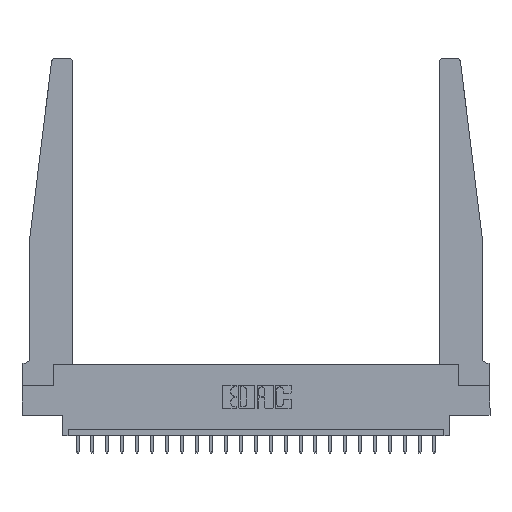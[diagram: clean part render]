
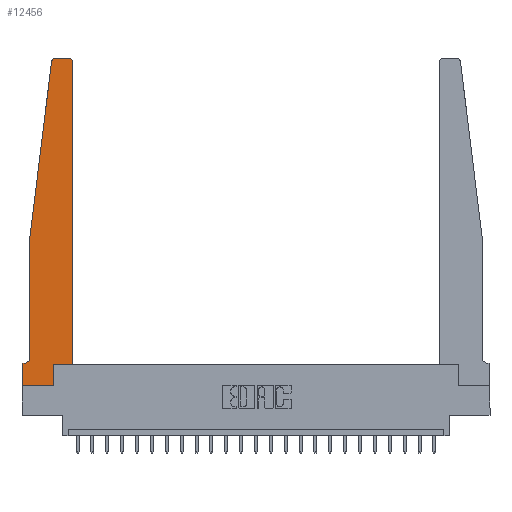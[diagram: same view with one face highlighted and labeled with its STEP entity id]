
A CAD part, top view. The second image highlights one B-rep face of the part: STEP entity #12456.
In plain terms, the highlighted planar face has unit normal (0, 0, 1).
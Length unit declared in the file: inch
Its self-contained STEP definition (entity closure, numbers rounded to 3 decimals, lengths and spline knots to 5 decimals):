
#195 = DIRECTION ( 'NONE',  ( 1., 0., 0. ) ) ;
#220 = CARTESIAN_POINT ( 'NONE',  ( 0.2605, 0.18, 0.37 ) ) ;
#1024 = VECTOR ( 'NONE', #21751, 39.37008 ) ;
#1156 = VECTOR ( 'NONE', #7244, 39.37008 ) ;
#1411 = VECTOR ( 'NONE', #16611, 39.37008 ) ;
#1470 = VERTEX_POINT ( 'NONE', #17604 ) ;
#1848 = DIRECTION ( 'NONE',  ( 0., 1., 0. ) ) ;
#1946 = LINE ( 'NONE', #5581, #20961 ) ;
#2087 = LINE ( 'NONE', #2330, #1411 ) ;
#2330 = CARTESIAN_POINT ( 'NONE',  ( 0.065, 0.1875, 0.37 ) ) ;
#2447 = CARTESIAN_POINT ( 'NONE',  ( 0., 0.1875, 0.37 ) ) ;
#2589 = ORIENTED_EDGE ( 'NONE', *, *, #8702, .T. ) ;
#2683 = VECTOR ( 'NONE', #5161, 39.37008 ) ;
#3617 = ORIENTED_EDGE ( 'NONE', *, *, #18605, .T. ) ;
#3707 = ORIENTED_EDGE ( 'NONE', *, *, #18947, .T. ) ;
#4768 = LINE ( 'NONE', #8746, #23114 ) ;
#5161 = DIRECTION ( 'NONE',  ( 0., -1., 0. ) ) ;
#5249 = CARTESIAN_POINT ( 'NONE',  ( 0., 0.1875, 0.37 ) ) ;
#5581 = CARTESIAN_POINT ( 'NONE',  ( 0.065, 1.25, 0.37 ) ) ;
#5660 = AXIS2_PLACEMENT_3D ( 'NONE', #9316, #14349, #16455 ) ;
#5969 = CIRCLE ( 'NONE', #7462, 0.03 ) ;
#6308 = CARTESIAN_POINT ( 'NONE',  ( 0.395, 2.75, 0.37 ) ) ;
#6386 = EDGE_CURVE ( 'NONE', #6647, #10797, #18316, .T. ) ;
#6418 = CARTESIAN_POINT ( 'NONE',  ( 0., 0., 0.37 ) ) ;
#6507 = DIRECTION ( 'NONE',  ( 0., 0., -1. ) ) ;
#6519 = DIRECTION ( 'NONE',  ( 1., 0., 0. ) ) ;
#6593 = CARTESIAN_POINT ( 'NONE',  ( 0.065, 1.25, 0.37 ) ) ;
#6647 = VERTEX_POINT ( 'NONE', #15839 ) ;
#6669 = ORIENTED_EDGE ( 'NONE', *, *, #12583, .T. ) ;
#7029 = EDGE_CURVE ( 'NONE', #15122, #15723, #5969, .T. ) ;
#7244 = DIRECTION ( 'NONE',  ( -1., 0., 0. ) ) ;
#7292 = CARTESIAN_POINT ( 'NONE',  ( 0.015, 0.1875, 0.37 ) ) ;
#7462 = AXIS2_PLACEMENT_3D ( 'NONE', #21162, #21394, #195 ) ;
#7508 = ORIENTED_EDGE ( 'NONE', *, *, #15579, .T. ) ;
#7677 = CARTESIAN_POINT ( 'NONE',  ( 0.2605, 0.18, 0.37 ) ) ;
#7858 = ORIENTED_EDGE ( 'NONE', *, *, #16598, .T. ) ;
#8171 = DIRECTION ( 'NONE',  ( -1., 0., 0. ) ) ;
#8194 = LINE ( 'NONE', #6418, #22127 ) ;
#8702 = EDGE_CURVE ( 'NONE', #14537, #20642, #16121, .T. ) ;
#8746 = CARTESIAN_POINT ( 'NONE',  ( 0.425, 0.18, 0.37 ) ) ;
#9017 = ORIENTED_EDGE ( 'NONE', *, *, #17111, .T. ) ;
#9165 = CARTESIAN_POINT ( 'NONE',  ( 0.27653, 2.75, 0.37 ) ) ;
#9316 = CARTESIAN_POINT ( 'NONE',  ( 0.395, 2.72, 0.37 ) ) ;
#9418 = DIRECTION ( 'NONE',  ( 0., 1., 0. ) ) ;
#9622 = CARTESIAN_POINT ( 'NONE',  ( 0.2605, 0., 0.37 ) ) ;
#9676 = VERTEX_POINT ( 'NONE', #6308 ) ;
#10520 = CIRCLE ( 'NONE', #5660, 0.03 ) ;
#10556 = CARTESIAN_POINT ( 'NONE',  ( 0.065, 1.25, 0.37 ) ) ;
#10649 = DIRECTION ( 'NONE',  ( 1., 0., 0. ) ) ;
#10797 = VERTEX_POINT ( 'NONE', #10815 ) ;
#10815 = CARTESIAN_POINT ( 'NONE',  ( 0.425, 2.72, 0.37 ) ) ;
#10895 = CARTESIAN_POINT ( 'NONE',  ( 0.25, 2.75, 0.37 ) ) ;
#10896 = CIRCLE ( 'NONE', #16109, 0.05 ) ;
#10981 = DIRECTION ( 'NONE',  ( -0.122, -0.992, 0. ) ) ;
#12015 = CARTESIAN_POINT ( 'NONE',  ( 0., 0., 0.37 ) ) ;
#12417 = DIRECTION ( 'NONE',  ( 0., 0., 1. ) ) ;
#12456 = ADVANCED_FACE ( 'NONE', ( #23060 ), #19537, .T. ) ;
#12573 = EDGE_CURVE ( 'NONE', #20124, #21087, #2087, .T. ) ;
#12583 = EDGE_CURVE ( 'NONE', #20642, #18800, #16260, .T. ) ;
#12707 = CARTESIAN_POINT ( 'NONE',  ( 0.425, 0.18, 0.37 ) ) ;
#12746 = CARTESIAN_POINT ( 'NONE',  ( 0., 0., 0.37 ) ) ;
#12835 = EDGE_CURVE ( 'NONE', #18800, #6647, #4768, .T. ) ;
#14349 = DIRECTION ( 'NONE',  ( 0., 0., 1. ) ) ;
#14537 = VERTEX_POINT ( 'NONE', #12015 ) ;
#15122 = VERTEX_POINT ( 'NONE', #9165 ) ;
#15149 = ORIENTED_EDGE ( 'NONE', *, *, #7029, .T. ) ;
#15181 = ORIENTED_EDGE ( 'NONE', *, *, #17052, .T. ) ;
#15251 = VECTOR ( 'NONE', #9418, 39.37008 ) ;
#15428 = CARTESIAN_POINT ( 'NONE',  ( 0.015, 0.2375, 0.37 ) ) ;
#15579 = EDGE_CURVE ( 'NONE', #15723, #17374, #1946, .T. ) ;
#15723 = VERTEX_POINT ( 'NONE', #17175 ) ;
#15839 = CARTESIAN_POINT ( 'NONE',  ( 0.425, 0.18, 0.37 ) ) ;
#16109 = AXIS2_PLACEMENT_3D ( 'NONE', #15428, #6507, #8171 ) ;
#16121 = LINE ( 'NONE', #12746, #1024 ) ;
#16260 = LINE ( 'NONE', #220, #21977 ) ;
#16455 = DIRECTION ( 'NONE',  ( 1., 0., 0. ) ) ;
#16598 = EDGE_CURVE ( 'NONE', #9676, #15122, #21780, .T. ) ;
#16611 = DIRECTION ( 'NONE',  ( -1., 0., 0. ) ) ;
#17052 = EDGE_CURVE ( 'NONE', #21087, #14537, #8194, .T. ) ;
#17111 = EDGE_CURVE ( 'NONE', #10797, #9676, #10520, .T. ) ;
#17175 = CARTESIAN_POINT ( 'NONE',  ( 0.24675, 2.72367, 0.37 ) ) ;
#17374 = VERTEX_POINT ( 'NONE', #6593 ) ;
#17604 = CARTESIAN_POINT ( 'NONE',  ( 0.065, 0.2375, 0.37 ) ) ;
#17614 = ORIENTED_EDGE ( 'NONE', *, *, #12573, .T. ) ;
#18316 = LINE ( 'NONE', #12707, #15251 ) ;
#18605 = EDGE_CURVE ( 'NONE', #1470, #20124, #10896, .T. ) ;
#18800 = VERTEX_POINT ( 'NONE', #7677 ) ;
#18947 = EDGE_CURVE ( 'NONE', #17374, #1470, #21318, .T. ) ;
#19537 = PLANE ( 'NONE',  #21612 ) ;
#20043 = ORIENTED_EDGE ( 'NONE', *, *, #12835, .T. ) ;
#20124 = VERTEX_POINT ( 'NONE', #7292 ) ;
#20257 = EDGE_LOOP ( 'NONE', ( #7858, #15149, #7508, #3707, #3617, #17614, #15181, #2589, #6669, #20043, #22549, #9017 ) ) ;
#20642 = VERTEX_POINT ( 'NONE', #9622 ) ;
#20961 = VECTOR ( 'NONE', #10981, 39.37008 ) ;
#21087 = VERTEX_POINT ( 'NONE', #2447 ) ;
#21162 = CARTESIAN_POINT ( 'NONE',  ( 0.27653, 2.72, 0.37 ) ) ;
#21318 = LINE ( 'NONE', #10556, #2683 ) ;
#21394 = DIRECTION ( 'NONE',  ( 0., 0., 1. ) ) ;
#21609 = DIRECTION ( 'NONE',  ( 0., -1., 0. ) ) ;
#21612 = AXIS2_PLACEMENT_3D ( 'NONE', #5249, #12417, #10649 ) ;
#21751 = DIRECTION ( 'NONE',  ( 1., 0., 0. ) ) ;
#21780 = LINE ( 'NONE', #10895, #1156 ) ;
#21977 = VECTOR ( 'NONE', #1848, 39.37008 ) ;
#22127 = VECTOR ( 'NONE', #21609, 39.37008 ) ;
#22549 = ORIENTED_EDGE ( 'NONE', *, *, #6386, .T. ) ;
#23060 = FACE_OUTER_BOUND ( 'NONE', #20257, .T. ) ;
#23114 = VECTOR ( 'NONE', #6519, 39.37008 ) ;
